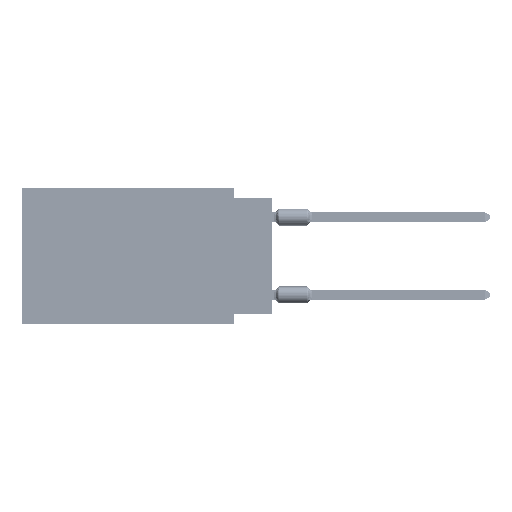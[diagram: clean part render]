
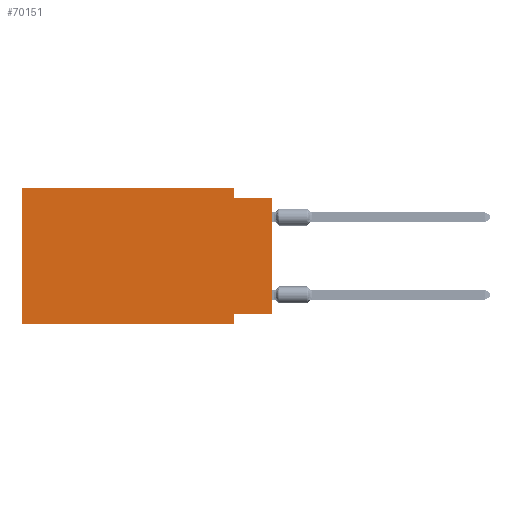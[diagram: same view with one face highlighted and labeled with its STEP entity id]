
A CAD part, left-side view. The second image highlights one B-rep face of the part: STEP entity #70151.
In plain terms, the highlighted planar face has unit normal (-1, 0, 0).
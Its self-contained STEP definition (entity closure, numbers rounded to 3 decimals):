
#676 = ORIENTED_EDGE ( 'NONE', *, *, #8498, .F. ) ;
#1196 = CARTESIAN_POINT ( 'NONE',  ( 0., 2.54, 0. ) ) ;
#4493 = VERTEX_POINT ( 'NONE', #55885 ) ;
#4818 = CARTESIAN_POINT ( 'NONE',  ( 0., 0., -8.255 ) ) ;
#8087 = LINE ( 'NONE', #40053, #35056 ) ;
#8498 = EDGE_CURVE ( 'NONE', #59970, #78971, #43419, .T. ) ;
#9710 = ORIENTED_EDGE ( 'NONE', *, *, #51409, .T. ) ;
#14211 = ORIENTED_EDGE ( 'NONE', *, *, #77597, .T. ) ;
#14851 = ORIENTED_EDGE ( 'NONE', *, *, #39300, .F. ) ;
#15783 = VERTEX_POINT ( 'NONE', #35385 ) ;
#16359 = VECTOR ( 'NONE', #62827, 1000. ) ;
#16408 = DIRECTION ( 'NONE',  ( 0., 0., -1. ) ) ;
#16767 = LINE ( 'NONE', #36176, #44725 ) ;
#17963 = CARTESIAN_POINT ( 'NONE',  ( 0., 16.383, 0. ) ) ;
#19640 = VECTOR ( 'NONE', #70607, 1000. ) ;
#20716 = LINE ( 'NONE', #71296, #62094 ) ;
#21252 = CARTESIAN_POINT ( 'NONE',  ( 0., 2.54, 0. ) ) ;
#22790 = ORIENTED_EDGE ( 'NONE', *, *, #36005, .F. ) ;
#23268 = VERTEX_POINT ( 'NONE', #54269 ) ;
#26350 = VERTEX_POINT ( 'NONE', #34055 ) ;
#27316 = LINE ( 'NONE', #21252, #19640 ) ;
#28694 = LINE ( 'NONE', #52975, #50107 ) ;
#29704 = ORIENTED_EDGE ( 'NONE', *, *, #50292, .F. ) ;
#34055 = CARTESIAN_POINT ( 'NONE',  ( 0., 16.383, -8.89 ) ) ;
#34233 = CARTESIAN_POINT ( 'NONE',  ( 0., 16.383, 0. ) ) ;
#34458 = DIRECTION ( 'NONE',  ( 0., -1., 0. ) ) ;
#35056 = VECTOR ( 'NONE', #51802, 1000. ) ;
#35385 = CARTESIAN_POINT ( 'NONE',  ( 0., 16.383, 0. ) ) ;
#36005 = EDGE_CURVE ( 'NONE', #4493, #61063, #20716, .T. ) ;
#36176 = CARTESIAN_POINT ( 'NONE',  ( 0., 0., 0. ) ) ;
#36403 = ORIENTED_EDGE ( 'NONE', *, *, #79394, .F. ) ;
#38260 = DIRECTION ( 'NONE',  ( 0., -1., 0. ) ) ;
#39300 = EDGE_CURVE ( 'NONE', #40792, #4493, #27316, .T. ) ;
#40053 = CARTESIAN_POINT ( 'NONE',  ( 0., 16.383, -8.89 ) ) ;
#40167 = ORIENTED_EDGE ( 'NONE', *, *, #44128, .F. ) ;
#40792 = VERTEX_POINT ( 'NONE', #1196 ) ;
#43419 = LINE ( 'NONE', #74969, #16359 ) ;
#44128 = EDGE_CURVE ( 'NONE', #15783, #40792, #69022, .T. ) ;
#44725 = VECTOR ( 'NONE', #66147, 1000. ) ;
#50107 = VECTOR ( 'NONE', #70377, 1000. ) ;
#50292 = EDGE_CURVE ( 'NONE', #26350, #15783, #55176, .T. ) ;
#51409 = EDGE_CURVE ( 'NONE', #26350, #23268, #8087, .T. ) ;
#51798 = AXIS2_PLACEMENT_3D ( 'NONE', #34233, #58907, #16408 ) ;
#51802 = DIRECTION ( 'NONE',  ( 0., -1., 0. ) ) ;
#52975 = CARTESIAN_POINT ( 'NONE',  ( 0., 2.54, -8.89 ) ) ;
#53252 = FACE_OUTER_BOUND ( 'NONE', #75155, .T. ) ;
#54269 = CARTESIAN_POINT ( 'NONE',  ( 0., 2.54, -8.89 ) ) ;
#55176 = LINE ( 'NONE', #17963, #74895 ) ;
#55885 = CARTESIAN_POINT ( 'NONE',  ( 0., 2.54, -0.635 ) ) ;
#58907 = DIRECTION ( 'NONE',  ( 1., 0., 0. ) ) ;
#59970 = VERTEX_POINT ( 'NONE', #4818 ) ;
#61063 = VERTEX_POINT ( 'NONE', #65567 ) ;
#62094 = VECTOR ( 'NONE', #34458, 1000. ) ;
#62827 = DIRECTION ( 'NONE',  ( 0., 1., 0. ) ) ;
#65567 = CARTESIAN_POINT ( 'NONE',  ( 0., 0., -0.635 ) ) ;
#66147 = DIRECTION ( 'NONE',  ( 0., 0., 1. ) ) ;
#69022 = LINE ( 'NONE', #73907, #79535 ) ;
#70151 = ADVANCED_FACE ( 'NONE', ( #53252 ), #71863, .F. ) ;
#70377 = DIRECTION ( 'NONE',  ( 0., 0., -1. ) ) ;
#70607 = DIRECTION ( 'NONE',  ( 0., 0., -1. ) ) ;
#71296 = CARTESIAN_POINT ( 'NONE',  ( 0., 0., -0.635 ) ) ;
#71863 = PLANE ( 'NONE',  #51798 ) ;
#73907 = CARTESIAN_POINT ( 'NONE',  ( 0., 16.383, 0. ) ) ;
#74895 = VECTOR ( 'NONE', #79857, 1000. ) ;
#74969 = CARTESIAN_POINT ( 'NONE',  ( 0., 0., -8.255 ) ) ;
#75155 = EDGE_LOOP ( 'NONE', ( #14211, #22790, #14851, #40167, #29704, #9710, #36403, #676 ) ) ;
#76532 = CARTESIAN_POINT ( 'NONE',  ( 0., 2.54, -8.255 ) ) ;
#77597 = EDGE_CURVE ( 'NONE', #59970, #61063, #16767, .T. ) ;
#78971 = VERTEX_POINT ( 'NONE', #76532 ) ;
#79394 = EDGE_CURVE ( 'NONE', #78971, #23268, #28694, .T. ) ;
#79535 = VECTOR ( 'NONE', #38260, 1000. ) ;
#79857 = DIRECTION ( 'NONE',  ( 0., 0., 1. ) ) ;
